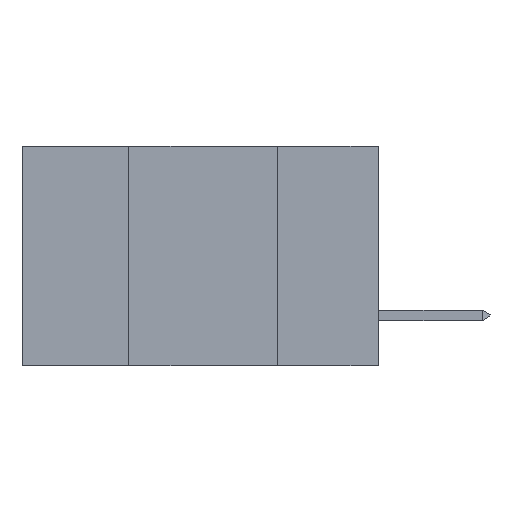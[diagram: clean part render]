
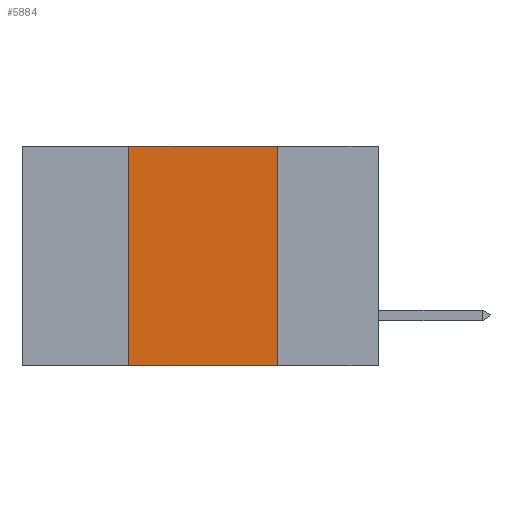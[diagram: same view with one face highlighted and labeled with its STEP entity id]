
A CAD part, left-side view. The second image highlights one B-rep face of the part: STEP entity #5884.
In plain terms, the highlighted planar face has unit normal (-1, 0, 0).
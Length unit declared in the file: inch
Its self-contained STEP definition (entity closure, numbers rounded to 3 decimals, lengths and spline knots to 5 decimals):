
#17 = EDGE_LOOP ( 'NONE', ( #20035, #20687, #24399, #7191 ) ) ;
#357 = CARTESIAN_POINT ( 'NONE',  ( 0., 0.42, 0. ) ) ;
#636 = VERTEX_POINT ( 'NONE', #16412 ) ;
#1190 = LINE ( 'NONE', #357, #10980 ) ;
#4574 = VERTEX_POINT ( 'NONE', #18951 ) ;
#4750 = DIRECTION ( 'NONE',  ( 0., 0., 1. ) ) ;
#5532 = VERTEX_POINT ( 'NONE', #14670 ) ;
#5604 = LINE ( 'NONE', #14732, #12743 ) ;
#5884 = ADVANCED_FACE ( 'NONE', ( #11845 ), #13212, .F. ) ;
#6373 = EDGE_CURVE ( 'NONE', #636, #21620, #5604, .T. ) ;
#7191 = ORIENTED_EDGE ( 'NONE', *, *, #19109, .T. ) ;
#9770 = LINE ( 'NONE', #12182, #23516 ) ;
#10731 = DIRECTION ( 'NONE',  ( 1., 0., 0. ) ) ;
#10980 = VECTOR ( 'NONE', #4750, 39.37008 ) ;
#11845 = FACE_OUTER_BOUND ( 'NONE', #17, .T. ) ;
#12092 = DIRECTION ( 'NONE',  ( 0., -1., 0. ) ) ;
#12182 = CARTESIAN_POINT ( 'NONE',  ( 0., 0.6, -0.37 ) ) ;
#12673 = DIRECTION ( 'NONE',  ( 0., -1., 0. ) ) ;
#12743 = VECTOR ( 'NONE', #12673, 39.37008 ) ;
#13212 = PLANE ( 'NONE',  #21674 ) ;
#14225 = CARTESIAN_POINT ( 'NONE',  ( 0., 0.17, 0. ) ) ;
#14670 = CARTESIAN_POINT ( 'NONE',  ( 0., 0.17, -0.37 ) ) ;
#14732 = CARTESIAN_POINT ( 'NONE',  ( 0., 0.6, 0. ) ) ;
#14926 = LINE ( 'NONE', #26889, #20144 ) ;
#15257 = EDGE_CURVE ( 'NONE', #4574, #636, #1190, .T. ) ;
#15450 = DIRECTION ( 'NONE',  ( 0., 0., -1. ) ) ;
#16412 = CARTESIAN_POINT ( 'NONE',  ( 0., 0.42, 0. ) ) ;
#18951 = CARTESIAN_POINT ( 'NONE',  ( 0., 0.42, -0.37 ) ) ;
#19109 = EDGE_CURVE ( 'NONE', #4574, #5532, #9770, .T. ) ;
#20035 = ORIENTED_EDGE ( 'NONE', *, *, #24361, .F. ) ;
#20144 = VECTOR ( 'NONE', #22964, 39.37008 ) ;
#20687 = ORIENTED_EDGE ( 'NONE', *, *, #6373, .F. ) ;
#21620 = VERTEX_POINT ( 'NONE', #14225 ) ;
#21674 = AXIS2_PLACEMENT_3D ( 'NONE', #23306, #10731, #15450 ) ;
#22964 = DIRECTION ( 'NONE',  ( 0., 0., -1. ) ) ;
#23306 = CARTESIAN_POINT ( 'NONE',  ( 0., 0.6, 0. ) ) ;
#23516 = VECTOR ( 'NONE', #12092, 39.37008 ) ;
#24361 = EDGE_CURVE ( 'NONE', #21620, #5532, #14926, .T. ) ;
#24399 = ORIENTED_EDGE ( 'NONE', *, *, #15257, .F. ) ;
#26889 = CARTESIAN_POINT ( 'NONE',  ( 0., 0.17, 0. ) ) ;
